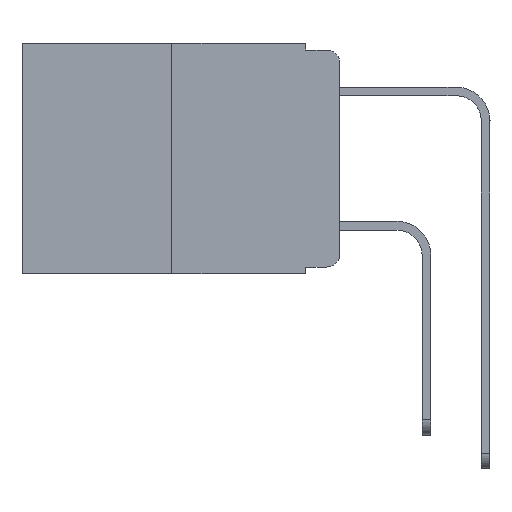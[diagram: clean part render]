
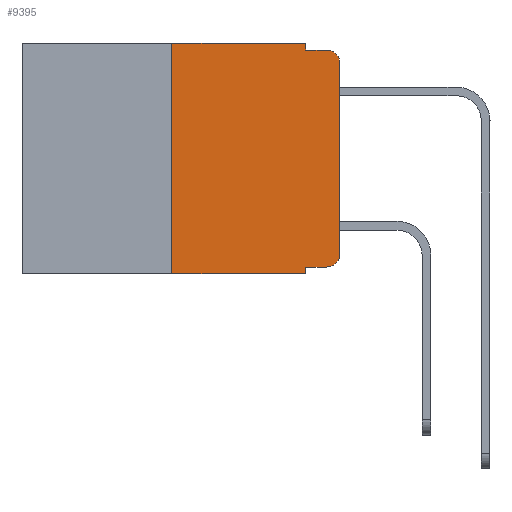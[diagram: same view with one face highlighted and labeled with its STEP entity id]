
A CAD part, left-side view. The second image highlights one B-rep face of the part: STEP entity #9395.
In plain terms, the highlighted planar face has unit normal (-1, 0, 0).
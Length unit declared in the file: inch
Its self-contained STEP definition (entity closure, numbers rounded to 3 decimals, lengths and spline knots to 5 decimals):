
#21 = ORIENTED_EDGE ( 'NONE', *, *, #7175, .T. ) ;
#119 = CARTESIAN_POINT ( 'NONE',  ( 0., 0.02, -0.333 ) ) ;
#207 = VECTOR ( 'NONE', #4482, 39.37008 ) ;
#363 = VERTEX_POINT ( 'NONE', #11467 ) ;
#431 = AXIS2_PLACEMENT_3D ( 'NONE', #3244, #10680, #4361 ) ;
#440 = VERTEX_POINT ( 'NONE', #10489 ) ;
#782 = CARTESIAN_POINT ( 'NONE',  ( 0., 0.051, 0. ) ) ;
#1019 = CARTESIAN_POINT ( 'NONE',  ( 0., 0.25, 0. ) ) ;
#1191 = VECTOR ( 'NONE', #1937, 39.37008 ) ;
#1217 = VERTEX_POINT ( 'NONE', #8322 ) ;
#1634 = VERTEX_POINT ( 'NONE', #4992 ) ;
#1937 = DIRECTION ( 'NONE',  ( 0., 0., -1. ) ) ;
#2220 = CARTESIAN_POINT ( 'NONE',  ( 0., 0.051, 0. ) ) ;
#2443 = EDGE_CURVE ( 'NONE', #5690, #440, #4012, .T. ) ;
#2816 = CARTESIAN_POINT ( 'NONE',  ( 0., 0.051, -0.333 ) ) ;
#2864 = ORIENTED_EDGE ( 'NONE', *, *, #11987, .F. ) ;
#3244 = CARTESIAN_POINT ( 'NONE',  ( 0., 0.02, -0.03 ) ) ;
#3939 = ORIENTED_EDGE ( 'NONE', *, *, #4049, .T. ) ;
#3998 = CARTESIAN_POINT ( 'NONE',  ( 0., 0.051, -0.333 ) ) ;
#3999 = LINE ( 'NONE', #9308, #6567 ) ;
#4012 = CIRCLE ( 'NONE', #8102, 0.02 ) ;
#4038 = VECTOR ( 'NONE', #4514, 39.37008 ) ;
#4049 = EDGE_CURVE ( 'NONE', #11879, #1634, #8671, .T. ) ;
#4290 = VERTEX_POINT ( 'NONE', #1019 ) ;
#4361 = DIRECTION ( 'NONE',  ( 0., 0., -1. ) ) ;
#4365 = CARTESIAN_POINT ( 'NONE',  ( 0., 0.25, -0.343 ) ) ;
#4482 = DIRECTION ( 'NONE',  ( 0., -1., 0. ) ) ;
#4514 = DIRECTION ( 'NONE',  ( 0., 0., 1. ) ) ;
#4624 = VECTOR ( 'NONE', #6586, 39.37008 ) ;
#4809 = DIRECTION ( 'NONE',  ( 0., -1., 0. ) ) ;
#4992 = CARTESIAN_POINT ( 'NONE',  ( 0., 0.051, -0.343 ) ) ;
#5113 = DIRECTION ( 'NONE',  ( 0., 0., -1. ) ) ;
#5128 = DIRECTION ( 'NONE',  ( 0., -1., 0. ) ) ;
#5550 = CARTESIAN_POINT ( 'NONE',  ( 0., 0.473, 0. ) ) ;
#5656 = LINE ( 'NONE', #3998, #11170 ) ;
#5690 = VERTEX_POINT ( 'NONE', #119 ) ;
#5723 = CARTESIAN_POINT ( 'NONE',  ( 0., 0., -0.03 ) ) ;
#5741 = EDGE_CURVE ( 'NONE', #440, #7324, #13235, .T. ) ;
#6134 = EDGE_LOOP ( 'NONE', ( #11334, #21, #12150, #12447, #13251, #9118, #3939, #2864, #8798, #6339 ) ) ;
#6339 = ORIENTED_EDGE ( 'NONE', *, *, #2443, .T. ) ;
#6567 = VECTOR ( 'NONE', #5113, 39.37008 ) ;
#6586 = DIRECTION ( 'NONE',  ( 0., 0., 1. ) ) ;
#6673 = DIRECTION ( 'NONE',  ( 1., 0., 0. ) ) ;
#7031 = CIRCLE ( 'NONE', #431, 0.02 ) ;
#7175 = EDGE_CURVE ( 'NONE', #7324, #363, #7031, .T. ) ;
#7250 = VERTEX_POINT ( 'NONE', #2220 ) ;
#7324 = VERTEX_POINT ( 'NONE', #5723 ) ;
#7478 = VECTOR ( 'NONE', #4809, 39.37008 ) ;
#7728 = CARTESIAN_POINT ( 'NONE',  ( 0., 0.473, -0.343 ) ) ;
#7872 = EDGE_CURVE ( 'NONE', #1217, #363, #9602, .T. ) ;
#8102 = AXIS2_PLACEMENT_3D ( 'NONE', #11862, #11834, #13208 ) ;
#8276 = FACE_OUTER_BOUND ( 'NONE', #6134, .T. ) ;
#8322 = CARTESIAN_POINT ( 'NONE',  ( 0., 0.051, -0.01 ) ) ;
#8671 = LINE ( 'NONE', #7728, #207 ) ;
#8725 = EDGE_CURVE ( 'NONE', #4290, #7250, #13216, .T. ) ;
#8798 = ORIENTED_EDGE ( 'NONE', *, *, #13317, .T. ) ;
#9118 = ORIENTED_EDGE ( 'NONE', *, *, #9940, .F. ) ;
#9243 = EDGE_CURVE ( 'NONE', #7250, #1217, #9888, .T. ) ;
#9308 = CARTESIAN_POINT ( 'NONE',  ( 0., 0.051, 0. ) ) ;
#9395 = ADVANCED_FACE ( 'NONE', ( #8276 ), #12808, .F. ) ;
#9602 = LINE ( 'NONE', #9785, #11993 ) ;
#9709 = LINE ( 'NONE', #9803, #4038 ) ;
#9785 = CARTESIAN_POINT ( 'NONE',  ( 0., 0.051, -0.01 ) ) ;
#9803 = CARTESIAN_POINT ( 'NONE',  ( 0., 0.25, 0. ) ) ;
#9888 = LINE ( 'NONE', #782, #1191 ) ;
#9940 = EDGE_CURVE ( 'NONE', #11879, #4290, #9709, .T. ) ;
#10489 = CARTESIAN_POINT ( 'NONE',  ( 0., 0., -0.313 ) ) ;
#10680 = DIRECTION ( 'NONE',  ( -1., 0., 0. ) ) ;
#10797 = DIRECTION ( 'NONE',  ( 0., -1., 0. ) ) ;
#11170 = VECTOR ( 'NONE', #5128, 39.37008 ) ;
#11334 = ORIENTED_EDGE ( 'NONE', *, *, #5741, .T. ) ;
#11467 = CARTESIAN_POINT ( 'NONE',  ( 0., 0.02, -0.01 ) ) ;
#11825 = CARTESIAN_POINT ( 'NONE',  ( 0., 0., 0. ) ) ;
#11834 = DIRECTION ( 'NONE',  ( -1., 0., 0. ) ) ;
#11862 = CARTESIAN_POINT ( 'NONE',  ( 0., 0.02, -0.313 ) ) ;
#11879 = VERTEX_POINT ( 'NONE', #4365 ) ;
#11987 = EDGE_CURVE ( 'NONE', #13836, #1634, #3999, .T. ) ;
#11993 = VECTOR ( 'NONE', #10797, 39.37008 ) ;
#12150 = ORIENTED_EDGE ( 'NONE', *, *, #7872, .F. ) ;
#12265 = AXIS2_PLACEMENT_3D ( 'NONE', #5550, #6673, #13843 ) ;
#12447 = ORIENTED_EDGE ( 'NONE', *, *, #9243, .F. ) ;
#12808 = PLANE ( 'NONE',  #12265 ) ;
#13073 = CARTESIAN_POINT ( 'NONE',  ( 0., 0.473, 0. ) ) ;
#13208 = DIRECTION ( 'NONE',  ( 0., 0., -1. ) ) ;
#13216 = LINE ( 'NONE', #13073, #7478 ) ;
#13235 = LINE ( 'NONE', #11825, #4624 ) ;
#13251 = ORIENTED_EDGE ( 'NONE', *, *, #8725, .F. ) ;
#13317 = EDGE_CURVE ( 'NONE', #13836, #5690, #5656, .T. ) ;
#13836 = VERTEX_POINT ( 'NONE', #2816 ) ;
#13843 = DIRECTION ( 'NONE',  ( 0., 0., -1. ) ) ;
